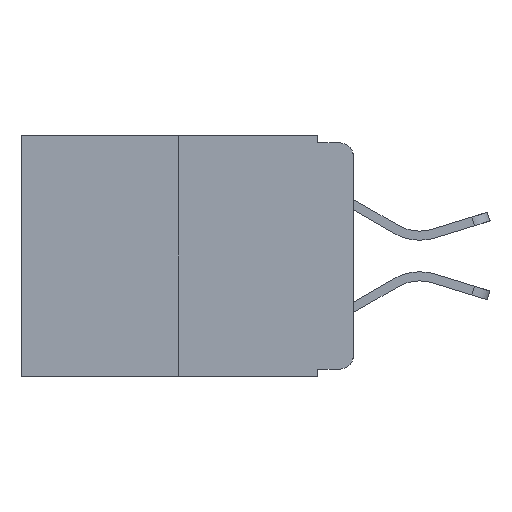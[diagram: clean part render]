
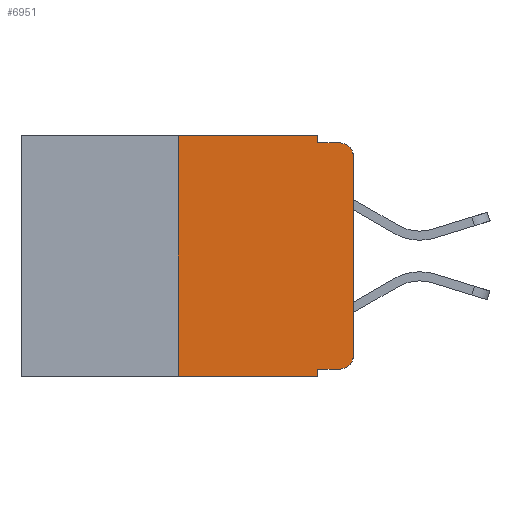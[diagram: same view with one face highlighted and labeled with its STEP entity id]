
A CAD part, left-side view. The second image highlights one B-rep face of the part: STEP entity #6951.
In plain terms, the highlighted planar face has unit normal (-1, 0, 0).
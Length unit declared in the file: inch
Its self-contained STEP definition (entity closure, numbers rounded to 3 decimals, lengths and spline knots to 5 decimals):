
#157 = DIRECTION ( 'NONE',  ( 0., -1., 0. ) ) ;
#197 = CARTESIAN_POINT ( 'NONE',  ( 0., 0.25, 0. ) ) ;
#331 = CIRCLE ( 'NONE', #11856, 0.02 ) ;
#425 = DIRECTION ( 'NONE',  ( 0., 0., -1. ) ) ;
#527 = PLANE ( 'NONE',  #11872 ) ;
#553 = CARTESIAN_POINT ( 'NONE',  ( 0., 0.051, -0.333 ) ) ;
#633 = VECTOR ( 'NONE', #157, 39.37008 ) ;
#1337 = VERTEX_POINT ( 'NONE', #197 ) ;
#1421 = ORIENTED_EDGE ( 'NONE', *, *, #17980, .F. ) ;
#1924 = CARTESIAN_POINT ( 'NONE',  ( 0., 0.051, -0.333 ) ) ;
#2114 = DIRECTION ( 'NONE',  ( 0., 0., 1. ) ) ;
#2145 = VECTOR ( 'NONE', #2114, 39.37008 ) ;
#2260 = DIRECTION ( 'NONE',  ( 0., -1., 0. ) ) ;
#2408 = LINE ( 'NONE', #553, #15400 ) ;
#3270 = ORIENTED_EDGE ( 'NONE', *, *, #6278, .T. ) ;
#3425 = EDGE_CURVE ( 'NONE', #4616, #1337, #7272, .T. ) ;
#3882 = VERTEX_POINT ( 'NONE', #1924 ) ;
#3956 = DIRECTION ( 'NONE',  ( 0., 0., -1. ) ) ;
#4022 = CARTESIAN_POINT ( 'NONE',  ( 0., 0.051, -0.01 ) ) ;
#4090 = AXIS2_PLACEMENT_3D ( 'NONE', #6109, #17880, #7772 ) ;
#4098 = ORIENTED_EDGE ( 'NONE', *, *, #10065, .F. ) ;
#4545 = CARTESIAN_POINT ( 'NONE',  ( 0., 0.051, -0.01 ) ) ;
#4616 = VERTEX_POINT ( 'NONE', #15807 ) ;
#5691 = CARTESIAN_POINT ( 'NONE',  ( 0., 0.051, -0.343 ) ) ;
#5869 = DIRECTION ( 'NONE',  ( -1., 0., 0. ) ) ;
#6109 = CARTESIAN_POINT ( 'NONE',  ( 0., 0.02, -0.03 ) ) ;
#6278 = EDGE_CURVE ( 'NONE', #13686, #17827, #20057, .T. ) ;
#6951 = ADVANCED_FACE ( 'NONE', ( #20919 ), #527, .F. ) ;
#6992 = VERTEX_POINT ( 'NONE', #4022 ) ;
#7184 = EDGE_LOOP ( 'NONE', ( #3270, #20123, #7757, #1421, #4098, #15754, #21737, #19911, #12063, #19151 ) ) ;
#7272 = LINE ( 'NONE', #9482, #11230 ) ;
#7746 = CIRCLE ( 'NONE', #4090, 0.02 ) ;
#7748 = CARTESIAN_POINT ( 'NONE',  ( 0., 0., -0.313 ) ) ;
#7757 = ORIENTED_EDGE ( 'NONE', *, *, #11451, .F. ) ;
#7772 = DIRECTION ( 'NONE',  ( 0., 0., -1. ) ) ;
#8189 = CARTESIAN_POINT ( 'NONE',  ( 0., 0.02, -0.333 ) ) ;
#8195 = VERTEX_POINT ( 'NONE', #5691 ) ;
#8592 = CARTESIAN_POINT ( 'NONE',  ( 0., 0.473, -0.343 ) ) ;
#9428 = VECTOR ( 'NONE', #16343, 39.37008 ) ;
#9482 = CARTESIAN_POINT ( 'NONE',  ( 0., 0.25, 0. ) ) ;
#9645 = CARTESIAN_POINT ( 'NONE',  ( 0., 0.02, -0.01 ) ) ;
#9917 = LINE ( 'NONE', #11232, #18363 ) ;
#10010 = LINE ( 'NONE', #20972, #18447 ) ;
#10065 = EDGE_CURVE ( 'NONE', #1337, #19809, #10010, .T. ) ;
#10507 = CARTESIAN_POINT ( 'NONE',  ( 0., 0., -0.03 ) ) ;
#11000 = DIRECTION ( 'NONE',  ( 0., -1., 0. ) ) ;
#11230 = VECTOR ( 'NONE', #21221, 39.37008 ) ;
#11232 = CARTESIAN_POINT ( 'NONE',  ( 0., 0.051, 0. ) ) ;
#11451 = EDGE_CURVE ( 'NONE', #6992, #14816, #18391, .T. ) ;
#11856 = AXIS2_PLACEMENT_3D ( 'NONE', #15987, #5869, #17646 ) ;
#11872 = AXIS2_PLACEMENT_3D ( 'NONE', #12368, #14075, #3956 ) ;
#12063 = ORIENTED_EDGE ( 'NONE', *, *, #14542, .T. ) ;
#12249 = CARTESIAN_POINT ( 'NONE',  ( 0., 0.051, 0. ) ) ;
#12368 = CARTESIAN_POINT ( 'NONE',  ( 0., 0.473, 0. ) ) ;
#12940 = DIRECTION ( 'NONE',  ( 0., 0., -1. ) ) ;
#12959 = EDGE_CURVE ( 'NONE', #17827, #14816, #7746, .T. ) ;
#13353 = EDGE_CURVE ( 'NONE', #4616, #8195, #18589, .T. ) ;
#13686 = VERTEX_POINT ( 'NONE', #7748 ) ;
#13872 = VERTEX_POINT ( 'NONE', #8189 ) ;
#14075 = DIRECTION ( 'NONE',  ( 1., 0., 0. ) ) ;
#14542 = EDGE_CURVE ( 'NONE', #3882, #13872, #2408, .T. ) ;
#14816 = VERTEX_POINT ( 'NONE', #9645 ) ;
#15322 = VECTOR ( 'NONE', #425, 39.37008 ) ;
#15400 = VECTOR ( 'NONE', #2260, 39.37008 ) ;
#15754 = ORIENTED_EDGE ( 'NONE', *, *, #3425, .F. ) ;
#15807 = CARTESIAN_POINT ( 'NONE',  ( 0., 0.25, -0.343 ) ) ;
#15907 = CARTESIAN_POINT ( 'NONE',  ( 0., 0.051, 0. ) ) ;
#15987 = CARTESIAN_POINT ( 'NONE',  ( 0., 0.02, -0.313 ) ) ;
#16333 = EDGE_CURVE ( 'NONE', #3882, #8195, #19717, .T. ) ;
#16343 = DIRECTION ( 'NONE',  ( 0., -1., 0. ) ) ;
#17646 = DIRECTION ( 'NONE',  ( 0., 0., -1. ) ) ;
#17827 = VERTEX_POINT ( 'NONE', #10507 ) ;
#17880 = DIRECTION ( 'NONE',  ( -1., 0., 0. ) ) ;
#17980 = EDGE_CURVE ( 'NONE', #19809, #6992, #9917, .T. ) ;
#18363 = VECTOR ( 'NONE', #12940, 39.37008 ) ;
#18391 = LINE ( 'NONE', #4545, #9428 ) ;
#18447 = VECTOR ( 'NONE', #11000, 39.37008 ) ;
#18589 = LINE ( 'NONE', #8592, #633 ) ;
#19151 = ORIENTED_EDGE ( 'NONE', *, *, #21644, .T. ) ;
#19717 = LINE ( 'NONE', #12249, #15322 ) ;
#19809 = VERTEX_POINT ( 'NONE', #15907 ) ;
#19911 = ORIENTED_EDGE ( 'NONE', *, *, #16333, .F. ) ;
#20057 = LINE ( 'NONE', #20582, #2145 ) ;
#20123 = ORIENTED_EDGE ( 'NONE', *, *, #12959, .T. ) ;
#20582 = CARTESIAN_POINT ( 'NONE',  ( 0., 0., 0. ) ) ;
#20919 = FACE_OUTER_BOUND ( 'NONE', #7184, .T. ) ;
#20972 = CARTESIAN_POINT ( 'NONE',  ( 0., 0.473, 0. ) ) ;
#21221 = DIRECTION ( 'NONE',  ( 0., 0., 1. ) ) ;
#21644 = EDGE_CURVE ( 'NONE', #13872, #13686, #331, .T. ) ;
#21737 = ORIENTED_EDGE ( 'NONE', *, *, #13353, .T. ) ;
